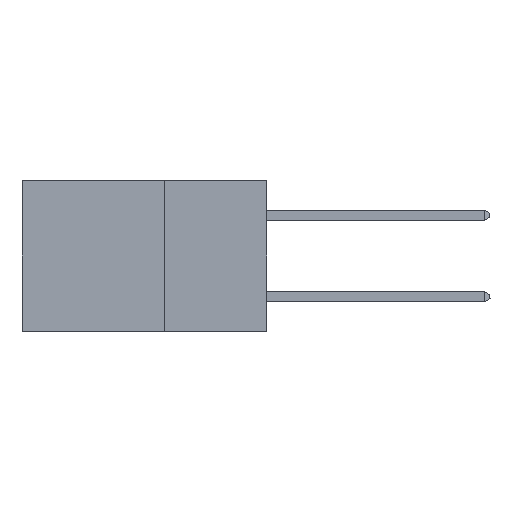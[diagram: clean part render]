
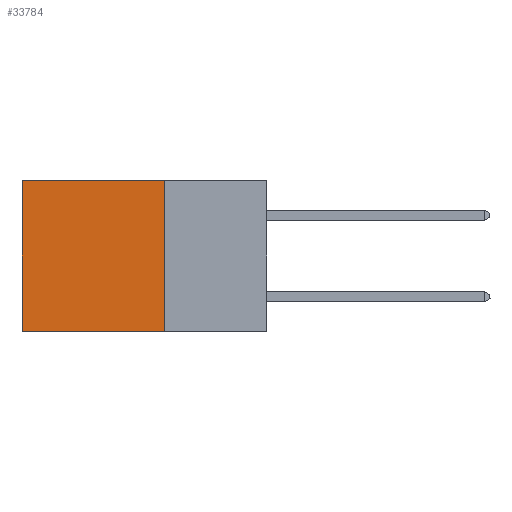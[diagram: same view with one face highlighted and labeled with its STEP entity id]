
A CAD part, left-side view. The second image highlights one B-rep face of the part: STEP entity #33784.
In plain terms, the highlighted planar face has unit normal (-1, 0, 0).
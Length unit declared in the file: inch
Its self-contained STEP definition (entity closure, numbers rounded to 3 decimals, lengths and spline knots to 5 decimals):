
#299 = VECTOR ( 'NONE', #16330, 39.37008 ) ;
#2160 = CARTESIAN_POINT ( 'NONE',  ( 0.2875, 0.6, 0. ) ) ;
#2761 = ORIENTED_EDGE ( 'NONE', *, *, #15411, .T. ) ;
#4576 = CARTESIAN_POINT ( 'NONE',  ( 0.2875, 0.6, -0.37 ) ) ;
#6265 = LINE ( 'NONE', #29528, #14139 ) ;
#6692 = CARTESIAN_POINT ( 'NONE',  ( 0.2875, 0.25, 0. ) ) ;
#7552 = EDGE_LOOP ( 'NONE', ( #2761, #13690, #16440, #32010 ) ) ;
#8548 = DIRECTION ( 'NONE',  ( 0., 0., -1. ) ) ;
#9790 = VERTEX_POINT ( 'NONE', #11080 ) ;
#11080 = CARTESIAN_POINT ( 'NONE',  ( 0.2875, 0.25, -0.37 ) ) ;
#11389 = LINE ( 'NONE', #2160, #299 ) ;
#12567 = EDGE_CURVE ( 'NONE', #24620, #9790, #26816, .T. ) ;
#13690 = ORIENTED_EDGE ( 'NONE', *, *, #36478, .F. ) ;
#14139 = VECTOR ( 'NONE', #35617, 39.37008 ) ;
#14435 = DIRECTION ( 'NONE',  ( 1., 0., 0. ) ) ;
#14585 = VECTOR ( 'NONE', #21513, 39.37008 ) ;
#15411 = EDGE_CURVE ( 'NONE', #23001, #16569, #11389, .T. ) ;
#16322 = DIRECTION ( 'NONE',  ( 0., 0., -1. ) ) ;
#16330 = DIRECTION ( 'NONE',  ( 0., 0., -1. ) ) ;
#16440 = ORIENTED_EDGE ( 'NONE', *, *, #12567, .F. ) ;
#16569 = VERTEX_POINT ( 'NONE', #4576 ) ;
#17365 = LINE ( 'NONE', #6692, #14585 ) ;
#19035 = VECTOR ( 'NONE', #16322, 39.37008 ) ;
#20522 = PLANE ( 'NONE',  #26468 ) ;
#21513 = DIRECTION ( 'NONE',  ( 0., 1., 0. ) ) ;
#22250 = CARTESIAN_POINT ( 'NONE',  ( 0.2875, 0.25, 0. ) ) ;
#23001 = VERTEX_POINT ( 'NONE', #25343 ) ;
#23212 = CARTESIAN_POINT ( 'NONE',  ( 0.2875, 0.25, 0. ) ) ;
#24620 = VERTEX_POINT ( 'NONE', #27863 ) ;
#25343 = CARTESIAN_POINT ( 'NONE',  ( 0.2875, 0.6, 0. ) ) ;
#26468 = AXIS2_PLACEMENT_3D ( 'NONE', #23212, #14435, #8548 ) ;
#26707 = FACE_OUTER_BOUND ( 'NONE', #7552, .T. ) ;
#26816 = LINE ( 'NONE', #22250, #19035 ) ;
#27863 = CARTESIAN_POINT ( 'NONE',  ( 0.2875, 0.25, 0. ) ) ;
#29446 = EDGE_CURVE ( 'NONE', #24620, #23001, #17365, .T. ) ;
#29528 = CARTESIAN_POINT ( 'NONE',  ( 0.2875, 0.25, -0.37 ) ) ;
#32010 = ORIENTED_EDGE ( 'NONE', *, *, #29446, .T. ) ;
#33784 = ADVANCED_FACE ( 'NONE', ( #26707 ), #20522, .F. ) ;
#35617 = DIRECTION ( 'NONE',  ( 0., 1., 0. ) ) ;
#36478 = EDGE_CURVE ( 'NONE', #9790, #16569, #6265, .T. ) ;
